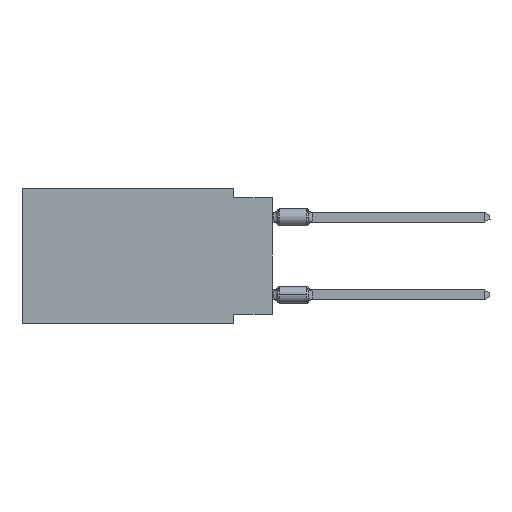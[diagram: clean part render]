
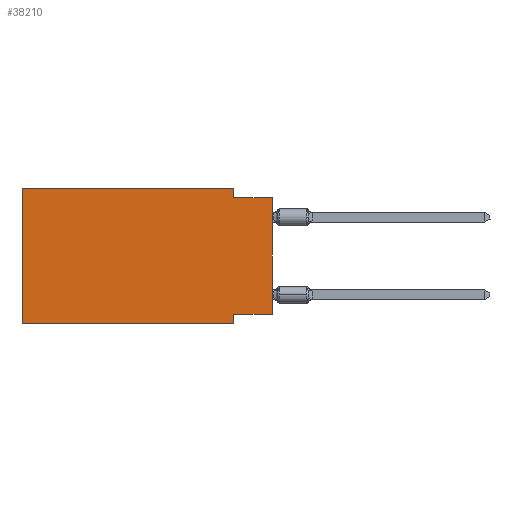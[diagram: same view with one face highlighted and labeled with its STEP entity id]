
A CAD part, left-side view. The second image highlights one B-rep face of the part: STEP entity #38210.
In plain terms, the highlighted planar face has unit normal (-1, 0, 0).
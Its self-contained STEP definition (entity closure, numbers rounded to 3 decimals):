
#147 = EDGE_LOOP ( 'NONE', ( #4779, #8240, #40392, #14545, #35299, #30240, #3323, #1208 ) ) ;
#1208 = ORIENTED_EDGE ( 'NONE', *, *, #38044, .F. ) ;
#2480 = LINE ( 'NONE', #28177, #38964 ) ;
#3210 = VECTOR ( 'NONE', #32265, 1000. ) ;
#3323 = ORIENTED_EDGE ( 'NONE', *, *, #27203, .F. ) ;
#4617 = LINE ( 'NONE', #27802, #32009 ) ;
#4779 = ORIENTED_EDGE ( 'NONE', *, *, #19322, .T. ) ;
#4907 = VERTEX_POINT ( 'NONE', #27821 ) ;
#5028 = DIRECTION ( 'NONE',  ( 0., 0., -1. ) ) ;
#8214 = CARTESIAN_POINT ( 'NONE',  ( 0., 16.383, -8.89 ) ) ;
#8240 = ORIENTED_EDGE ( 'NONE', *, *, #19467, .F. ) ;
#8816 = CARTESIAN_POINT ( 'NONE',  ( 0., 0., -8.255 ) ) ;
#11182 = VERTEX_POINT ( 'NONE', #35891 ) ;
#13608 = VECTOR ( 'NONE', #41219, 1000. ) ;
#14177 = VECTOR ( 'NONE', #17766, 1000. ) ;
#14545 = ORIENTED_EDGE ( 'NONE', *, *, #40694, .F. ) ;
#14849 = VERTEX_POINT ( 'NONE', #22364 ) ;
#15699 = LINE ( 'NONE', #28447, #13608 ) ;
#16264 = LINE ( 'NONE', #28185, #23463 ) ;
#16671 = CARTESIAN_POINT ( 'NONE',  ( 0., 16.383, 0. ) ) ;
#16924 = AXIS2_PLACEMENT_3D ( 'NONE', #16671, #36307, #27081 ) ;
#17766 = DIRECTION ( 'NONE',  ( 0., 0., -1. ) ) ;
#17943 = DIRECTION ( 'NONE',  ( 0., 1., 0. ) ) ;
#18427 = VERTEX_POINT ( 'NONE', #30771 ) ;
#19322 = EDGE_CURVE ( 'NONE', #30187, #14849, #27894, .T. ) ;
#19467 = EDGE_CURVE ( 'NONE', #11182, #14849, #23054, .T. ) ;
#19534 = CARTESIAN_POINT ( 'NONE',  ( 0., 0., -0.635 ) ) ;
#19614 = CARTESIAN_POINT ( 'NONE',  ( 0., 16.383, 0. ) ) ;
#22262 = CARTESIAN_POINT ( 'NONE',  ( 0., 2.54, -8.255 ) ) ;
#22364 = CARTESIAN_POINT ( 'NONE',  ( 0., 0., -0.635 ) ) ;
#22449 = VERTEX_POINT ( 'NONE', #22262 ) ;
#23054 = LINE ( 'NONE', #19534, #3210 ) ;
#23463 = VECTOR ( 'NONE', #25256, 1000. ) ;
#23545 = FACE_OUTER_BOUND ( 'NONE', #147, .T. ) ;
#24034 = LINE ( 'NONE', #26759, #14177 ) ;
#25256 = DIRECTION ( 'NONE',  ( 0., -1., 0. ) ) ;
#25656 = DIRECTION ( 'NONE',  ( 0., 0., 1. ) ) ;
#26759 = CARTESIAN_POINT ( 'NONE',  ( 0., 2.54, -8.89 ) ) ;
#27081 = DIRECTION ( 'NONE',  ( 0., 0., -1. ) ) ;
#27203 = EDGE_CURVE ( 'NONE', #22449, #18427, #24034, .T. ) ;
#27205 = VECTOR ( 'NONE', #27478, 1000. ) ;
#27478 = DIRECTION ( 'NONE',  ( 0., 0., 1. ) ) ;
#27802 = CARTESIAN_POINT ( 'NONE',  ( 0., 2.54, 0. ) ) ;
#27821 = CARTESIAN_POINT ( 'NONE',  ( 0., 2.54, 0. ) ) ;
#27894 = LINE ( 'NONE', #40250, #27205 ) ;
#28177 = CARTESIAN_POINT ( 'NONE',  ( 0., 0., -8.255 ) ) ;
#28185 = CARTESIAN_POINT ( 'NONE',  ( 0., 16.383, -8.89 ) ) ;
#28447 = CARTESIAN_POINT ( 'NONE',  ( 0., 16.383, 0. ) ) ;
#30187 = VERTEX_POINT ( 'NONE', #8816 ) ;
#30226 = PLANE ( 'NONE',  #16924 ) ;
#30240 = ORIENTED_EDGE ( 'NONE', *, *, #35610, .T. ) ;
#30552 = VERTEX_POINT ( 'NONE', #31758 ) ;
#30771 = CARTESIAN_POINT ( 'NONE',  ( 0., 2.54, -8.89 ) ) ;
#31631 = EDGE_CURVE ( 'NONE', #4907, #11182, #4617, .T. ) ;
#31758 = CARTESIAN_POINT ( 'NONE',  ( 0., 16.383, 0. ) ) ;
#32009 = VECTOR ( 'NONE', #5028, 1000. ) ;
#32145 = LINE ( 'NONE', #19614, #32923 ) ;
#32265 = DIRECTION ( 'NONE',  ( 0., -1., 0. ) ) ;
#32829 = VERTEX_POINT ( 'NONE', #8214 ) ;
#32923 = VECTOR ( 'NONE', #25656, 1000. ) ;
#35299 = ORIENTED_EDGE ( 'NONE', *, *, #38099, .F. ) ;
#35610 = EDGE_CURVE ( 'NONE', #32829, #18427, #16264, .T. ) ;
#35891 = CARTESIAN_POINT ( 'NONE',  ( 0., 2.54, -0.635 ) ) ;
#36307 = DIRECTION ( 'NONE',  ( 1., 0., 0. ) ) ;
#38044 = EDGE_CURVE ( 'NONE', #30187, #22449, #2480, .T. ) ;
#38099 = EDGE_CURVE ( 'NONE', #32829, #30552, #32145, .T. ) ;
#38210 = ADVANCED_FACE ( 'NONE', ( #23545 ), #30226, .F. ) ;
#38964 = VECTOR ( 'NONE', #17943, 1000. ) ;
#40250 = CARTESIAN_POINT ( 'NONE',  ( 0., 0., 0. ) ) ;
#40392 = ORIENTED_EDGE ( 'NONE', *, *, #31631, .F. ) ;
#40694 = EDGE_CURVE ( 'NONE', #30552, #4907, #15699, .T. ) ;
#41219 = DIRECTION ( 'NONE',  ( 0., -1., 0. ) ) ;
